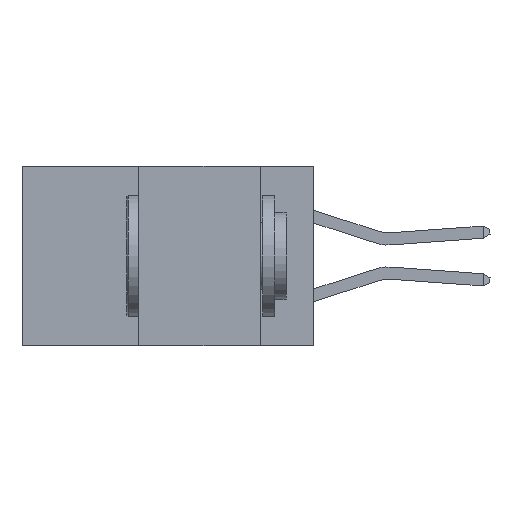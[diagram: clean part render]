
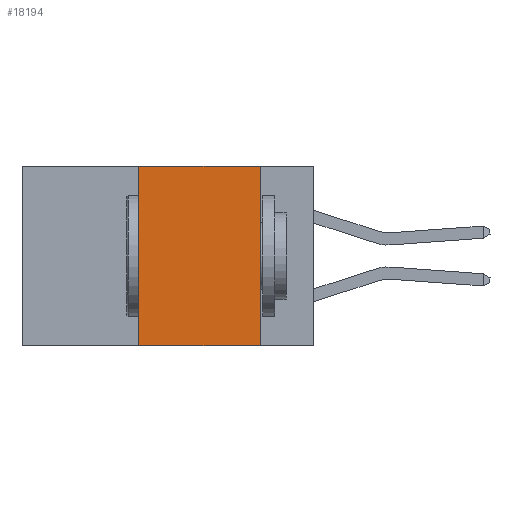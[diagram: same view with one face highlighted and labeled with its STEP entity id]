
A CAD part, left-side view. The second image highlights one B-rep face of the part: STEP entity #18194.
In plain terms, the highlighted planar face has unit normal (-1, 0, 0).
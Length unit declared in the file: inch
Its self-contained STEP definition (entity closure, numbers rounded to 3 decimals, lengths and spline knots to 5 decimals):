
#245 = VECTOR ( 'NONE', #3074, 39.37008 ) ;
#514 = CARTESIAN_POINT ( 'NONE',  ( 0., 0.6, 0. ) ) ;
#2132 = ORIENTED_EDGE ( 'NONE', *, *, #8943, .F. ) ;
#2307 = PLANE ( 'NONE',  #33871 ) ;
#3074 = DIRECTION ( 'NONE',  ( 0., 0., -1. ) ) ;
#3618 = LINE ( 'NONE', #9448, #245 ) ;
#4146 = EDGE_CURVE ( 'NONE', #28757, #35053, #3618, .T. ) ;
#5403 = DIRECTION ( 'NONE',  ( 1., 0., 0. ) ) ;
#8943 = EDGE_CURVE ( 'NONE', #13421, #31811, #30131, .T. ) ;
#9356 = CARTESIAN_POINT ( 'NONE',  ( 0., 0.11, 0. ) ) ;
#9448 = CARTESIAN_POINT ( 'NONE',  ( 0., 0.11, 0. ) ) ;
#9533 = CARTESIAN_POINT ( 'NONE',  ( 0., 0.11, -0.37 ) ) ;
#10620 = ORIENTED_EDGE ( 'NONE', *, *, #19832, .T. ) ;
#12331 = VECTOR ( 'NONE', #30816, 39.37008 ) ;
#13421 = VERTEX_POINT ( 'NONE', #39759 ) ;
#13744 = DIRECTION ( 'NONE',  ( 0., 0., 1. ) ) ;
#14056 = ORIENTED_EDGE ( 'NONE', *, *, #4146, .F. ) ;
#14316 = LINE ( 'NONE', #39254, #12331 ) ;
#15050 = ORIENTED_EDGE ( 'NONE', *, *, #27524, .F. ) ;
#16629 = DIRECTION ( 'NONE',  ( 0., -1., 0. ) ) ;
#18194 = ADVANCED_FACE ( 'NONE', ( #38314 ), #2307, .F. ) ;
#18367 = EDGE_LOOP ( 'NONE', ( #14056, #15050, #2132, #10620 ) ) ;
#19832 = EDGE_CURVE ( 'NONE', #13421, #35053, #14316, .T. ) ;
#21361 = VECTOR ( 'NONE', #13744, 39.37008 ) ;
#22315 = CARTESIAN_POINT ( 'NONE',  ( 0., 0.36, 0. ) ) ;
#26248 = CARTESIAN_POINT ( 'NONE',  ( 0., 0.36, 0. ) ) ;
#27524 = EDGE_CURVE ( 'NONE', #31811, #28757, #32473, .T. ) ;
#28757 = VERTEX_POINT ( 'NONE', #9356 ) ;
#30131 = LINE ( 'NONE', #26248, #21361 ) ;
#30317 = CARTESIAN_POINT ( 'NONE',  ( 0., 0.6, 0. ) ) ;
#30816 = DIRECTION ( 'NONE',  ( 0., -1., 0. ) ) ;
#31473 = VECTOR ( 'NONE', #16629, 39.37008 ) ;
#31811 = VERTEX_POINT ( 'NONE', #22315 ) ;
#32473 = LINE ( 'NONE', #514, #31473 ) ;
#33871 = AXIS2_PLACEMENT_3D ( 'NONE', #30317, #5403, #39945 ) ;
#35053 = VERTEX_POINT ( 'NONE', #9533 ) ;
#38314 = FACE_OUTER_BOUND ( 'NONE', #18367, .T. ) ;
#39254 = CARTESIAN_POINT ( 'NONE',  ( 0., 0.6, -0.37 ) ) ;
#39759 = CARTESIAN_POINT ( 'NONE',  ( 0., 0.36, -0.37 ) ) ;
#39945 = DIRECTION ( 'NONE',  ( 0., 0., -1. ) ) ;
